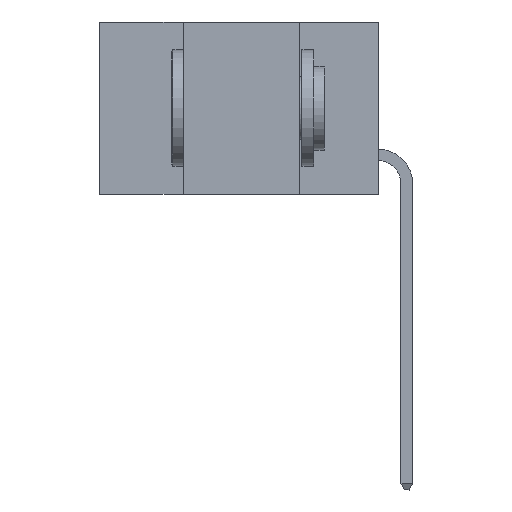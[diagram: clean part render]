
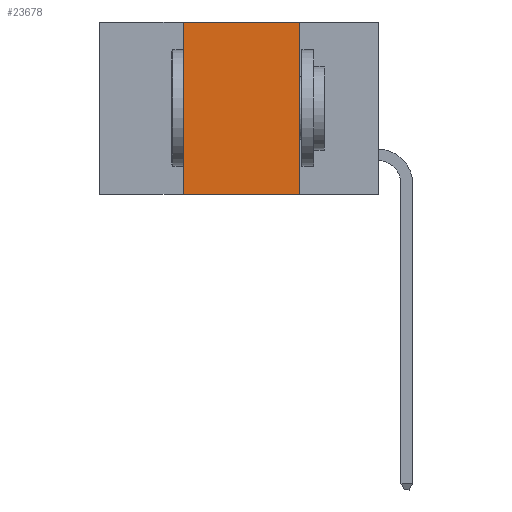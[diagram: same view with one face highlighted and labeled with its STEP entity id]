
A CAD part, left-side view. The second image highlights one B-rep face of the part: STEP entity #23678.
In plain terms, the highlighted planar face has unit normal (-1, 0, 0).
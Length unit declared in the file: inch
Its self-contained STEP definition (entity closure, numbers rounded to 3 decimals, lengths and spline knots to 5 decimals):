
#375 = DIRECTION ( 'NONE',  ( 0., -1., 0. ) ) ;
#1149 = CARTESIAN_POINT ( 'NONE',  ( 0., 0.6, 0. ) ) ;
#2133 = EDGE_LOOP ( 'NONE', ( #19535, #19280, #22741, #25128 ) ) ;
#3405 = PLANE ( 'NONE',  #18703 ) ;
#3749 = EDGE_CURVE ( 'NONE', #18458, #11565, #25720, .T. ) ;
#7546 = LINE ( 'NONE', #14582, #28169 ) ;
#8720 = VERTEX_POINT ( 'NONE', #13983 ) ;
#11183 = CARTESIAN_POINT ( 'NONE',  ( 0., 0.42, -0.37 ) ) ;
#11565 = VERTEX_POINT ( 'NONE', #24223 ) ;
#11598 = VECTOR ( 'NONE', #18338, 39.37008 ) ;
#12133 = CARTESIAN_POINT ( 'NONE',  ( 0., 0.42, 0. ) ) ;
#12212 = EDGE_CURVE ( 'NONE', #25593, #8720, #25675, .T. ) ;
#13983 = CARTESIAN_POINT ( 'NONE',  ( 0., 0.17, 0. ) ) ;
#14408 = CARTESIAN_POINT ( 'NONE',  ( 0., 0.6, 0. ) ) ;
#14582 = CARTESIAN_POINT ( 'NONE',  ( 0., 0.17, 0. ) ) ;
#15803 = VECTOR ( 'NONE', #21286, 39.37008 ) ;
#17053 = FACE_OUTER_BOUND ( 'NONE', #2133, .T. ) ;
#17303 = EDGE_CURVE ( 'NONE', #8720, #11565, #7546, .T. ) ;
#18158 = VECTOR ( 'NONE', #375, 39.37008 ) ;
#18338 = DIRECTION ( 'NONE',  ( 0., -1., 0. ) ) ;
#18458 = VERTEX_POINT ( 'NONE', #11183 ) ;
#18703 = AXIS2_PLACEMENT_3D ( 'NONE', #1149, #19161, #21872 ) ;
#19161 = DIRECTION ( 'NONE',  ( 1., 0., 0. ) ) ;
#19280 = ORIENTED_EDGE ( 'NONE', *, *, #12212, .F. ) ;
#19494 = EDGE_CURVE ( 'NONE', #18458, #25593, #25794, .T. ) ;
#19535 = ORIENTED_EDGE ( 'NONE', *, *, #17303, .F. ) ;
#21286 = DIRECTION ( 'NONE',  ( 0., 0., 1. ) ) ;
#21872 = DIRECTION ( 'NONE',  ( 0., 0., -1. ) ) ;
#22741 = ORIENTED_EDGE ( 'NONE', *, *, #19494, .F. ) ;
#23678 = ADVANCED_FACE ( 'NONE', ( #17053 ), #3405, .F. ) ;
#23759 = CARTESIAN_POINT ( 'NONE',  ( 0., 0.6, -0.37 ) ) ;
#24223 = CARTESIAN_POINT ( 'NONE',  ( 0., 0.17, -0.37 ) ) ;
#25128 = ORIENTED_EDGE ( 'NONE', *, *, #3749, .T. ) ;
#25593 = VERTEX_POINT ( 'NONE', #28409 ) ;
#25675 = LINE ( 'NONE', #14408, #11598 ) ;
#25720 = LINE ( 'NONE', #23759, #18158 ) ;
#25794 = LINE ( 'NONE', #12133, #15803 ) ;
#27965 = DIRECTION ( 'NONE',  ( 0., 0., -1. ) ) ;
#28169 = VECTOR ( 'NONE', #27965, 39.37008 ) ;
#28409 = CARTESIAN_POINT ( 'NONE',  ( 0., 0.42, 0. ) ) ;
